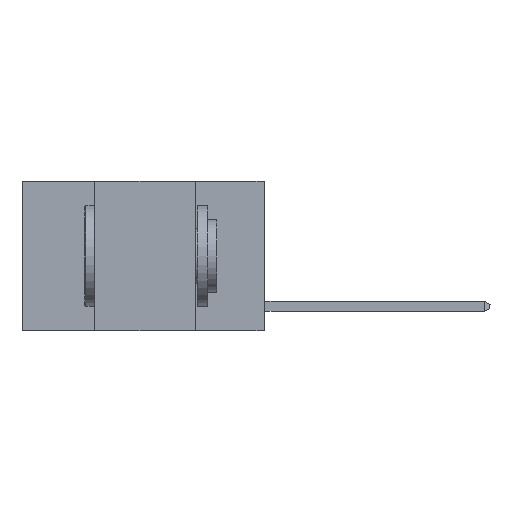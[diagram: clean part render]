
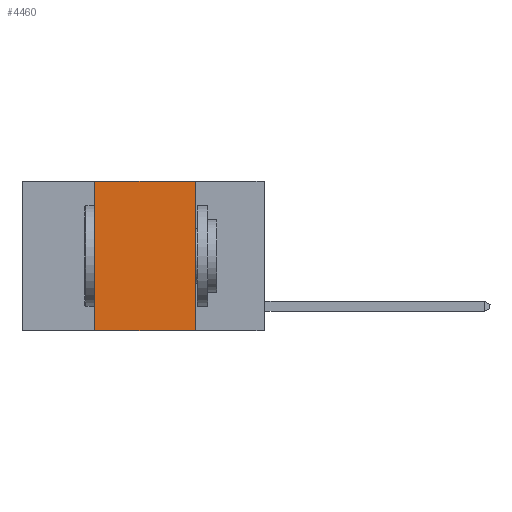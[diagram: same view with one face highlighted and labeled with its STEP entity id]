
A CAD part, left-side view. The second image highlights one B-rep face of the part: STEP entity #4460.
In plain terms, the highlighted planar face has unit normal (-1, 0, 0).
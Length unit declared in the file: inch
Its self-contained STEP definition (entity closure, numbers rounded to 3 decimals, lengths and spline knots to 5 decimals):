
#19 = AXIS2_PLACEMENT_3D ( 'NONE', #5093, #9197, #32 ) ;
#32 = DIRECTION ( 'NONE',  ( 0., 0., -1. ) ) ;
#72 = VECTOR ( 'NONE', #12186, 39.37008 ) ;
#1467 = VERTEX_POINT ( 'NONE', #1491 ) ;
#1491 = CARTESIAN_POINT ( 'NONE',  ( 0., 0.42, -0.37 ) ) ;
#1837 = EDGE_CURVE ( 'NONE', #1467, #9037, #7245, .T. ) ;
#2014 = PLANE ( 'NONE',  #19 ) ;
#2651 = VERTEX_POINT ( 'NONE', #12591 ) ;
#2847 = ORIENTED_EDGE ( 'NONE', *, *, #1837, .F. ) ;
#3261 = ORIENTED_EDGE ( 'NONE', *, *, #12581, .F. ) ;
#4271 = LINE ( 'NONE', #7297, #4369 ) ;
#4369 = VECTOR ( 'NONE', #5202, 39.37008 ) ;
#4460 = ADVANCED_FACE ( 'NONE', ( #11193 ), #2014, .F. ) ;
#4779 = CARTESIAN_POINT ( 'NONE',  ( 0., 0.17, 0. ) ) ;
#5093 = CARTESIAN_POINT ( 'NONE',  ( 0., 0.6, 0. ) ) ;
#5202 = DIRECTION ( 'NONE',  ( 0., -1., 0. ) ) ;
#7245 = LINE ( 'NONE', #9259, #7701 ) ;
#7297 = CARTESIAN_POINT ( 'NONE',  ( 0., 0.6, -0.37 ) ) ;
#7701 = VECTOR ( 'NONE', #11312, 39.37008 ) ;
#7891 = LINE ( 'NONE', #9838, #9534 ) ;
#8285 = EDGE_CURVE ( 'NONE', #12734, #2651, #9270, .T. ) ;
#9037 = VERTEX_POINT ( 'NONE', #10775 ) ;
#9197 = DIRECTION ( 'NONE',  ( 1., 0., 0. ) ) ;
#9259 = CARTESIAN_POINT ( 'NONE',  ( 0., 0.42, 0. ) ) ;
#9270 = LINE ( 'NONE', #4779, #72 ) ;
#9534 = VECTOR ( 'NONE', #10960, 39.37008 ) ;
#9838 = CARTESIAN_POINT ( 'NONE',  ( 0., 0.6, 0. ) ) ;
#9977 = EDGE_LOOP ( 'NONE', ( #11014, #3261, #2847, #12269 ) ) ;
#10775 = CARTESIAN_POINT ( 'NONE',  ( 0., 0.42, 0. ) ) ;
#10960 = DIRECTION ( 'NONE',  ( 0., -1., 0. ) ) ;
#11014 = ORIENTED_EDGE ( 'NONE', *, *, #8285, .F. ) ;
#11193 = FACE_OUTER_BOUND ( 'NONE', #9977, .T. ) ;
#11221 = CARTESIAN_POINT ( 'NONE',  ( 0., 0.17, 0. ) ) ;
#11312 = DIRECTION ( 'NONE',  ( 0., 0., 1. ) ) ;
#12186 = DIRECTION ( 'NONE',  ( 0., 0., -1. ) ) ;
#12262 = EDGE_CURVE ( 'NONE', #1467, #2651, #4271, .T. ) ;
#12269 = ORIENTED_EDGE ( 'NONE', *, *, #12262, .T. ) ;
#12581 = EDGE_CURVE ( 'NONE', #9037, #12734, #7891, .T. ) ;
#12591 = CARTESIAN_POINT ( 'NONE',  ( 0., 0.17, -0.37 ) ) ;
#12734 = VERTEX_POINT ( 'NONE', #11221 ) ;
